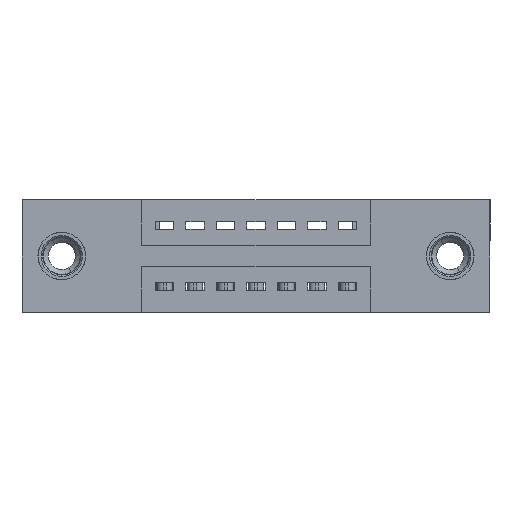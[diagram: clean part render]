
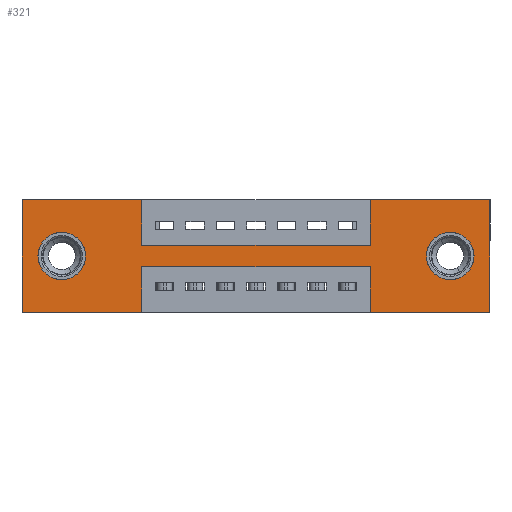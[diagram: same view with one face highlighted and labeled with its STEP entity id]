
A CAD part, front view. The second image highlights one B-rep face of the part: STEP entity #321.
In plain terms, the highlighted planar face has unit normal (0, -1, 0).
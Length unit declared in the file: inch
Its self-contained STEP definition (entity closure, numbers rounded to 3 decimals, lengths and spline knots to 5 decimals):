
#130 = EDGE_CURVE ( 'NONE', #9314, #1617, #2510, .T. ) ;
#193 = VERTEX_POINT ( 'NONE', #7750 ) ;
#321 = ADVANCED_FACE ( 'NONE', ( #9012, #13156, #5999 ), #6294, .T. ) ;
#485 = VECTOR ( 'NONE', #6115, 39.37008 ) ;
#528 = CARTESIAN_POINT ( 'NONE',  ( 1.535, 0., 0. ) ) ;
#693 = ORIENTED_EDGE ( 'NONE', *, *, #8276, .F. ) ;
#885 = CARTESIAN_POINT ( 'NONE',  ( 1.535, 0., 0. ) ) ;
#897 = DIRECTION ( 'NONE',  ( 0., 0., 1. ) ) ;
#995 = CARTESIAN_POINT ( 'NONE',  ( 0., 0., 0. ) ) ;
#1015 = CARTESIAN_POINT ( 'NONE',  ( 0.3925, 0., 0. ) ) ;
#1334 = VECTOR ( 'NONE', #897, 39.37008 ) ;
#1617 = VERTEX_POINT ( 'NONE', #8787 ) ;
#1674 = ORIENTED_EDGE ( 'NONE', *, *, #7718, .F. ) ;
#1685 = ORIENTED_EDGE ( 'NONE', *, *, #5059, .T. ) ;
#1902 = VECTOR ( 'NONE', #13911, 39.37008 ) ;
#1938 = CARTESIAN_POINT ( 'NONE',  ( 1.1425, 0., 0. ) ) ;
#1975 = VECTOR ( 'NONE', #10571, 39.37008 ) ;
#2146 = CARTESIAN_POINT ( 'NONE',  ( 1.405, 0., -0.107 ) ) ;
#2226 = VECTOR ( 'NONE', #14040, 39.37008 ) ;
#2510 = LINE ( 'NONE', #10336, #13163 ) ;
#2522 = CARTESIAN_POINT ( 'NONE',  ( 0.13, 0., -0.107 ) ) ;
#2562 = ORIENTED_EDGE ( 'NONE', *, *, #8124, .T. ) ;
#2781 = DIRECTION ( 'NONE',  ( 0., 0., -1. ) ) ;
#2923 = LINE ( 'NONE', #1938, #1334 ) ;
#3227 = EDGE_CURVE ( 'NONE', #5857, #9314, #6648, .T. ) ;
#3320 = EDGE_CURVE ( 'NONE', #3780, #5857, #7734, .T. ) ;
#3486 = DIRECTION ( 'NONE',  ( 0., 0., -1. ) ) ;
#3535 = EDGE_LOOP ( 'NONE', ( #1685, #4616 ) ) ;
#3596 = CARTESIAN_POINT ( 'NONE',  ( 1.535, 0., -0.37 ) ) ;
#3669 = CARTESIAN_POINT ( 'NONE',  ( 0.3925, 0., -0.15 ) ) ;
#3674 = CIRCLE ( 'NONE', #6855, 0.078 ) ;
#3780 = VERTEX_POINT ( 'NONE', #3596 ) ;
#3798 = CIRCLE ( 'NONE', #4565, 0.078 ) ;
#4113 = CARTESIAN_POINT ( 'NONE',  ( 1.405, 0., -0.185 ) ) ;
#4380 = CARTESIAN_POINT ( 'NONE',  ( 1.405, 0., -0.185 ) ) ;
#4418 = CIRCLE ( 'NONE', #6660, 0.078 ) ;
#4504 = DIRECTION ( 'NONE',  ( 0., 0., -1. ) ) ;
#4508 = LINE ( 'NONE', #5869, #2226 ) ;
#4565 = AXIS2_PLACEMENT_3D ( 'NONE', #4380, #7768, #9945 ) ;
#4566 = ORIENTED_EDGE ( 'NONE', *, *, #10101, .F. ) ;
#4616 = ORIENTED_EDGE ( 'NONE', *, *, #10218, .T. ) ;
#4665 = LINE ( 'NONE', #13737, #13392 ) ;
#4695 = ORIENTED_EDGE ( 'NONE', *, *, #7640, .F. ) ;
#4718 = DIRECTION ( 'NONE',  ( -1., 0., 0. ) ) ;
#4927 = EDGE_CURVE ( 'NONE', #8182, #193, #12390, .T. ) ;
#5007 = DIRECTION ( 'NONE',  ( -1., 0., 0. ) ) ;
#5054 = VERTEX_POINT ( 'NONE', #2146 ) ;
#5059 = EDGE_CURVE ( 'NONE', #10598, #6925, #6828, .T. ) ;
#5097 = ORIENTED_EDGE ( 'NONE', *, *, #3227, .F. ) ;
#5129 = DIRECTION ( 'NONE',  ( -1., 0., 0. ) ) ;
#5394 = DIRECTION ( 'NONE',  ( 0., 0., 1. ) ) ;
#5555 = CARTESIAN_POINT ( 'NONE',  ( 0.13, 0., -0.185 ) ) ;
#5703 = EDGE_CURVE ( 'NONE', #5054, #5921, #3674, .T. ) ;
#5752 = CARTESIAN_POINT ( 'NONE',  ( 1.1425, 0., -0.15 ) ) ;
#5857 = VERTEX_POINT ( 'NONE', #6141 ) ;
#5869 = CARTESIAN_POINT ( 'NONE',  ( 0., 0., 0. ) ) ;
#5921 = VERTEX_POINT ( 'NONE', #11954 ) ;
#5976 = EDGE_LOOP ( 'NONE', ( #693, #11967, #5097, #13192, #4566, #1674, #4695, #11023, #11157, #12011, #9749, #14255 ) ) ;
#5999 = FACE_OUTER_BOUND ( 'NONE', #5976, .T. ) ;
#6115 = DIRECTION ( 'NONE',  ( 0., 0., 1. ) ) ;
#6141 = CARTESIAN_POINT ( 'NONE',  ( 1.1425, 0., -0.37 ) ) ;
#6205 = VERTEX_POINT ( 'NONE', #8808 ) ;
#6244 = DIRECTION ( 'NONE',  ( 0., -1., 0. ) ) ;
#6294 = PLANE ( 'NONE',  #11778 ) ;
#6644 = DIRECTION ( 'NONE',  ( 0., 1., 0. ) ) ;
#6648 = LINE ( 'NONE', #14329, #11641 ) ;
#6660 = AXIS2_PLACEMENT_3D ( 'NONE', #14388, #14335, #8789 ) ;
#6828 = CIRCLE ( 'NONE', #10190, 0.078 ) ;
#6855 = AXIS2_PLACEMENT_3D ( 'NONE', #4113, #12032, #10893 ) ;
#6925 = VERTEX_POINT ( 'NONE', #11792 ) ;
#7103 = VERTEX_POINT ( 'NONE', #13416 ) ;
#7185 = EDGE_CURVE ( 'NONE', #6205, #10484, #14338, .T. ) ;
#7220 = CARTESIAN_POINT ( 'NONE',  ( 0., 0., -0.37 ) ) ;
#7475 = EDGE_CURVE ( 'NONE', #7103, #6205, #4508, .T. ) ;
#7640 = EDGE_CURVE ( 'NONE', #11278, #10783, #2923, .T. ) ;
#7690 = CARTESIAN_POINT ( 'NONE',  ( 1.1425, 0., -0.22 ) ) ;
#7699 = LINE ( 'NONE', #3669, #1902 ) ;
#7718 = EDGE_CURVE ( 'NONE', #10783, #12943, #13050, .T. ) ;
#7734 = LINE ( 'NONE', #7220, #11839 ) ;
#7750 = CARTESIAN_POINT ( 'NONE',  ( 0., 0., -0.37 ) ) ;
#7768 = DIRECTION ( 'NONE',  ( 0., 1., 0. ) ) ;
#7967 = CARTESIAN_POINT ( 'NONE',  ( 0.3925, 0., -0.37 ) ) ;
#8124 = EDGE_CURVE ( 'NONE', #5921, #5054, #3798, .T. ) ;
#8182 = VERTEX_POINT ( 'NONE', #7967 ) ;
#8276 = EDGE_CURVE ( 'NONE', #1617, #8182, #4665, .T. ) ;
#8525 = CARTESIAN_POINT ( 'NONE',  ( 0., 0., -0.37 ) ) ;
#8764 = DIRECTION ( 'NONE',  ( 0., 0., 1. ) ) ;
#8787 = CARTESIAN_POINT ( 'NONE',  ( 0.3925, 0., -0.22 ) ) ;
#8789 = DIRECTION ( 'NONE',  ( 0., 0., 1. ) ) ;
#8808 = CARTESIAN_POINT ( 'NONE',  ( 0.3925, 0., 0. ) ) ;
#8905 = VECTOR ( 'NONE', #12325, 39.37008 ) ;
#9012 = FACE_BOUND ( 'NONE', #14228, .T. ) ;
#9151 = CARTESIAN_POINT ( 'NONE',  ( 0.3925, 0., -0.15 ) ) ;
#9314 = VERTEX_POINT ( 'NONE', #7690 ) ;
#9509 = VECTOR ( 'NONE', #5007, 39.37008 ) ;
#9749 = ORIENTED_EDGE ( 'NONE', *, *, #13861, .F. ) ;
#9834 = VECTOR ( 'NONE', #4504, 39.37008 ) ;
#9945 = DIRECTION ( 'NONE',  ( 0., 0., -1. ) ) ;
#10101 = EDGE_CURVE ( 'NONE', #12943, #3780, #14397, .T. ) ;
#10190 = AXIS2_PLACEMENT_3D ( 'NONE', #5555, #6644, #8764 ) ;
#10218 = EDGE_CURVE ( 'NONE', #6925, #10598, #4418, .T. ) ;
#10336 = CARTESIAN_POINT ( 'NONE',  ( 0.3925, 0., -0.22 ) ) ;
#10484 = VERTEX_POINT ( 'NONE', #9151 ) ;
#10571 = DIRECTION ( 'NONE',  ( 0., 0., -1. ) ) ;
#10598 = VERTEX_POINT ( 'NONE', #2522 ) ;
#10783 = VERTEX_POINT ( 'NONE', #11904 ) ;
#10893 = DIRECTION ( 'NONE',  ( 0., 0., -1. ) ) ;
#11023 = ORIENTED_EDGE ( 'NONE', *, *, #13724, .F. ) ;
#11157 = ORIENTED_EDGE ( 'NONE', *, *, #7185, .F. ) ;
#11278 = VERTEX_POINT ( 'NONE', #5752 ) ;
#11641 = VECTOR ( 'NONE', #5394, 39.37008 ) ;
#11778 = AXIS2_PLACEMENT_3D ( 'NONE', #8525, #6244, #2781 ) ;
#11779 = CARTESIAN_POINT ( 'NONE',  ( 0., 0., -0.37 ) ) ;
#11792 = CARTESIAN_POINT ( 'NONE',  ( 0.13, 0., -0.263 ) ) ;
#11839 = VECTOR ( 'NONE', #5129, 39.37008 ) ;
#11904 = CARTESIAN_POINT ( 'NONE',  ( 1.1425, 0., 0. ) ) ;
#11954 = CARTESIAN_POINT ( 'NONE',  ( 1.405, 0., -0.263 ) ) ;
#11967 = ORIENTED_EDGE ( 'NONE', *, *, #130, .F. ) ;
#12011 = ORIENTED_EDGE ( 'NONE', *, *, #7475, .F. ) ;
#12032 = DIRECTION ( 'NONE',  ( 0., 1., 0. ) ) ;
#12325 = DIRECTION ( 'NONE',  ( 1., 0., 0. ) ) ;
#12390 = LINE ( 'NONE', #11779, #9509 ) ;
#12524 = ORIENTED_EDGE ( 'NONE', *, *, #5703, .T. ) ;
#12710 = LINE ( 'NONE', #14005, #485 ) ;
#12943 = VERTEX_POINT ( 'NONE', #885 ) ;
#13050 = LINE ( 'NONE', #995, #8905 ) ;
#13156 = FACE_BOUND ( 'NONE', #3535, .T. ) ;
#13163 = VECTOR ( 'NONE', #4718, 39.37008 ) ;
#13192 = ORIENTED_EDGE ( 'NONE', *, *, #3320, .F. ) ;
#13392 = VECTOR ( 'NONE', #3486, 39.37008 ) ;
#13416 = CARTESIAN_POINT ( 'NONE',  ( 0., 0., 0. ) ) ;
#13724 = EDGE_CURVE ( 'NONE', #10484, #11278, #7699, .T. ) ;
#13737 = CARTESIAN_POINT ( 'NONE',  ( 0.3925, 0., -0.37 ) ) ;
#13861 = EDGE_CURVE ( 'NONE', #193, #7103, #12710, .T. ) ;
#13911 = DIRECTION ( 'NONE',  ( 1., 0., 0. ) ) ;
#14005 = CARTESIAN_POINT ( 'NONE',  ( 0., 0., 0. ) ) ;
#14040 = DIRECTION ( 'NONE',  ( 1., 0., 0. ) ) ;
#14228 = EDGE_LOOP ( 'NONE', ( #12524, #2562 ) ) ;
#14255 = ORIENTED_EDGE ( 'NONE', *, *, #4927, .F. ) ;
#14329 = CARTESIAN_POINT ( 'NONE',  ( 1.1425, 0., -0.37 ) ) ;
#14335 = DIRECTION ( 'NONE',  ( 0., 1., 0. ) ) ;
#14338 = LINE ( 'NONE', #1015, #9834 ) ;
#14388 = CARTESIAN_POINT ( 'NONE',  ( 0.13, 0., -0.185 ) ) ;
#14397 = LINE ( 'NONE', #528, #1975 ) ;
